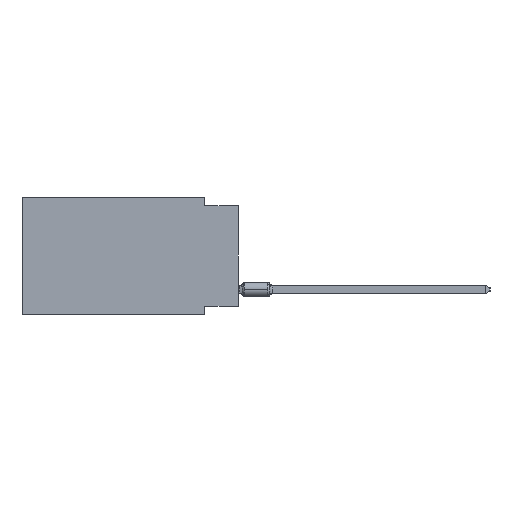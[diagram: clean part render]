
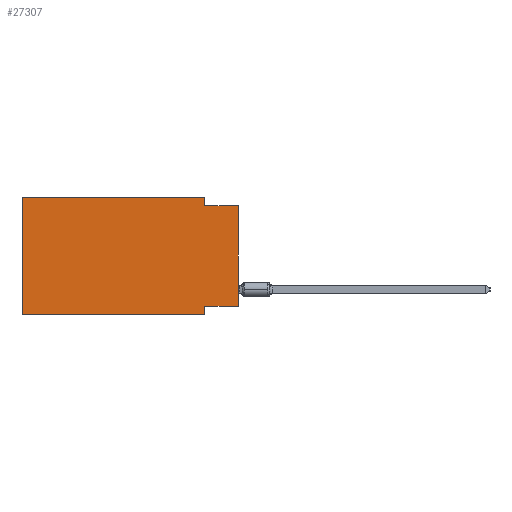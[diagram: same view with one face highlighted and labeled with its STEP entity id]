
A CAD part, left-side view. The second image highlights one B-rep face of the part: STEP entity #27307.
In plain terms, the highlighted planar face has unit normal (-1, 0, 0).
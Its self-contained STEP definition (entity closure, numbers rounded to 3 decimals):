
#141 = CARTESIAN_POINT ( 'NONE',  ( 0., 16.383, -8.89 ) ) ;
#3581 = EDGE_LOOP ( 'NONE', ( #19877, #63130, #53026, #41175, #52068, #8408, #48426, #60151 ) ) ;
#4387 = LINE ( 'NONE', #61675, #51200 ) ;
#6661 = DIRECTION ( 'NONE',  ( 0., -1., 0. ) ) ;
#7453 = VERTEX_POINT ( 'NONE', #17496 ) ;
#7950 = CARTESIAN_POINT ( 'NONE',  ( 0., 0., -0.635 ) ) ;
#8408 = ORIENTED_EDGE ( 'NONE', *, *, #32910, .T. ) ;
#9879 = CARTESIAN_POINT ( 'NONE',  ( 0., 0., 0. ) ) ;
#11579 = DIRECTION ( 'NONE',  ( 0., 0., -1. ) ) ;
#11844 = VERTEX_POINT ( 'NONE', #52859 ) ;
#13001 = CARTESIAN_POINT ( 'NONE',  ( 0., 16.383, 0. ) ) ;
#13998 = LINE ( 'NONE', #9879, #27704 ) ;
#14119 = EDGE_CURVE ( 'NONE', #21658, #11844, #42773, .T. ) ;
#14176 = VECTOR ( 'NONE', #16687, 1000. ) ;
#15047 = EDGE_CURVE ( 'NONE', #56500, #38030, #65886, .T. ) ;
#15314 = VECTOR ( 'NONE', #17881, 1000. ) ;
#15938 = VECTOR ( 'NONE', #11579, 1000. ) ;
#16687 = DIRECTION ( 'NONE',  ( 0., -1., 0. ) ) ;
#17496 = CARTESIAN_POINT ( 'NONE',  ( 0., 2.54, -8.89 ) ) ;
#17881 = DIRECTION ( 'NONE',  ( 0., 1., 0. ) ) ;
#18990 = CARTESIAN_POINT ( 'NONE',  ( 0., 2.54, -0.635 ) ) ;
#19877 = ORIENTED_EDGE ( 'NONE', *, *, #24171, .T. ) ;
#20391 = VERTEX_POINT ( 'NONE', #18990 ) ;
#21658 = VERTEX_POINT ( 'NONE', #61198 ) ;
#21833 = CARTESIAN_POINT ( 'NONE',  ( 0., 16.383, 0. ) ) ;
#24171 = EDGE_CURVE ( 'NONE', #56500, #49351, #13998, .T. ) ;
#25121 = CARTESIAN_POINT ( 'NONE',  ( 0., 16.383, 0. ) ) ;
#25460 = FACE_OUTER_BOUND ( 'NONE', #3581, .T. ) ;
#26928 = LINE ( 'NONE', #64294, #40386 ) ;
#27307 = ADVANCED_FACE ( 'NONE', ( #25460 ), #51182, .F. ) ;
#27704 = VECTOR ( 'NONE', #56190, 1000. ) ;
#28893 = DIRECTION ( 'NONE',  ( 0., -1., 0. ) ) ;
#32177 = LINE ( 'NONE', #58581, #15938 ) ;
#32910 = EDGE_CURVE ( 'NONE', #66161, #7453, #26928, .T. ) ;
#34036 = LINE ( 'NONE', #7950, #50048 ) ;
#38030 = VERTEX_POINT ( 'NONE', #49042 ) ;
#39086 = LINE ( 'NONE', #13001, #60760 ) ;
#39304 = CARTESIAN_POINT ( 'NONE',  ( 0., 0., -0.635 ) ) ;
#39827 = CARTESIAN_POINT ( 'NONE',  ( 0., 0., -8.255 ) ) ;
#40386 = VECTOR ( 'NONE', #6661, 1000. ) ;
#40543 = EDGE_CURVE ( 'NONE', #66161, #21658, #39086, .T. ) ;
#41175 = ORIENTED_EDGE ( 'NONE', *, *, #14119, .F. ) ;
#42773 = LINE ( 'NONE', #21833, #14176 ) ;
#44993 = EDGE_CURVE ( 'NONE', #38030, #7453, #4387, .T. ) ;
#47573 = AXIS2_PLACEMENT_3D ( 'NONE', #25121, #62154, #66962 ) ;
#48426 = ORIENTED_EDGE ( 'NONE', *, *, #44993, .F. ) ;
#49042 = CARTESIAN_POINT ( 'NONE',  ( 0., 2.54, -8.255 ) ) ;
#49351 = VERTEX_POINT ( 'NONE', #39304 ) ;
#50048 = VECTOR ( 'NONE', #28893, 1000. ) ;
#51182 = PLANE ( 'NONE',  #47573 ) ;
#51200 = VECTOR ( 'NONE', #67516, 1000. ) ;
#52068 = ORIENTED_EDGE ( 'NONE', *, *, #40543, .F. ) ;
#52823 = EDGE_CURVE ( 'NONE', #11844, #20391, #32177, .T. ) ;
#52859 = CARTESIAN_POINT ( 'NONE',  ( 0., 2.54, 0. ) ) ;
#53026 = ORIENTED_EDGE ( 'NONE', *, *, #52823, .F. ) ;
#54845 = DIRECTION ( 'NONE',  ( 0., 0., 1. ) ) ;
#55930 = EDGE_CURVE ( 'NONE', #20391, #49351, #34036, .T. ) ;
#56190 = DIRECTION ( 'NONE',  ( 0., 0., 1. ) ) ;
#56500 = VERTEX_POINT ( 'NONE', #59528 ) ;
#58581 = CARTESIAN_POINT ( 'NONE',  ( 0., 2.54, 0. ) ) ;
#59528 = CARTESIAN_POINT ( 'NONE',  ( 0., 0., -8.255 ) ) ;
#60151 = ORIENTED_EDGE ( 'NONE', *, *, #15047, .F. ) ;
#60760 = VECTOR ( 'NONE', #54845, 1000. ) ;
#61198 = CARTESIAN_POINT ( 'NONE',  ( 0., 16.383, 0. ) ) ;
#61675 = CARTESIAN_POINT ( 'NONE',  ( 0., 2.54, -8.89 ) ) ;
#62154 = DIRECTION ( 'NONE',  ( 1., 0., 0. ) ) ;
#63130 = ORIENTED_EDGE ( 'NONE', *, *, #55930, .F. ) ;
#64294 = CARTESIAN_POINT ( 'NONE',  ( 0., 16.383, -8.89 ) ) ;
#65886 = LINE ( 'NONE', #39827, #15314 ) ;
#66161 = VERTEX_POINT ( 'NONE', #141 ) ;
#66962 = DIRECTION ( 'NONE',  ( 0., 0., -1. ) ) ;
#67516 = DIRECTION ( 'NONE',  ( 0., 0., -1. ) ) ;
